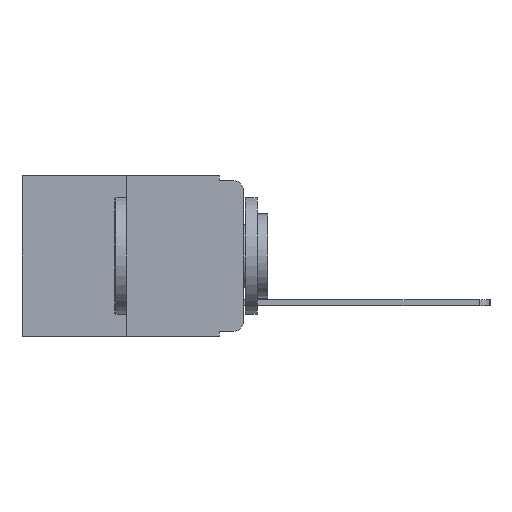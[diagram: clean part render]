
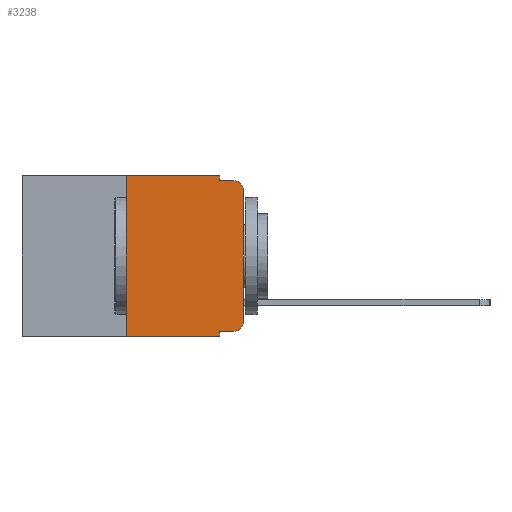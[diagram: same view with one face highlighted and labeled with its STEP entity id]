
A CAD part, left-side view. The second image highlights one B-rep face of the part: STEP entity #3238.
In plain terms, the highlighted planar face has unit normal (-1, 0, 0).
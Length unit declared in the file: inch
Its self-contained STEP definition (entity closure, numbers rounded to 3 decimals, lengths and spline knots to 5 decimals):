
#72 = ORIENTED_EDGE ( 'NONE', *, *, #2104, .F. ) ;
#92 = EDGE_CURVE ( 'NONE', #22968, #7479, #22821, .T. ) ;
#195 = VECTOR ( 'NONE', #9870, 39.37008 ) ;
#472 = DIRECTION ( 'NONE',  ( 0., -1., 0. ) ) ;
#510 = CIRCLE ( 'NONE', #16154, 0.02 ) ;
#915 = EDGE_CURVE ( 'NONE', #16615, #19250, #18439, .T. ) ;
#943 = CARTESIAN_POINT ( 'NONE',  ( 0., 0.25, 0. ) ) ;
#1352 = VERTEX_POINT ( 'NONE', #4210 ) ;
#1891 = AXIS2_PLACEMENT_3D ( 'NONE', #5693, #5776, #18304 ) ;
#2012 = ORIENTED_EDGE ( 'NONE', *, *, #2025, .T. ) ;
#2025 = EDGE_CURVE ( 'NONE', #11673, #21753, #6939, .T. ) ;
#2029 = EDGE_CURVE ( 'NONE', #21753, #4110, #510, .T. ) ;
#2096 = EDGE_CURVE ( 'NONE', #11606, #4110, #17285, .T. ) ;
#2104 = EDGE_CURVE ( 'NONE', #19250, #11606, #2763, .T. ) ;
#2208 = EDGE_CURVE ( 'NONE', #22968, #16615, #4902, .T. ) ;
#2303 = ORIENTED_EDGE ( 'NONE', *, *, #2434, .T. ) ;
#2334 = EDGE_CURVE ( 'NONE', #21268, #7479, #16415, .T. ) ;
#2406 = EDGE_CURVE ( 'NONE', #21268, #1352, #9529, .T. ) ;
#2434 = EDGE_CURVE ( 'NONE', #1352, #11673, #13143, .T. ) ;
#2763 = LINE ( 'NONE', #9090, #16729 ) ;
#3238 = ADVANCED_FACE ( 'NONE', ( #14453 ), #12986, .F. ) ;
#3280 = CARTESIAN_POINT ( 'NONE',  ( 0., 0.051, -0.333 ) ) ;
#4050 = CARTESIAN_POINT ( 'NONE',  ( 0., 0.051, -0.01 ) ) ;
#4110 = VERTEX_POINT ( 'NONE', #19022 ) ;
#4210 = CARTESIAN_POINT ( 'NONE',  ( 0., 0.02, -0.333 ) ) ;
#4368 = CARTESIAN_POINT ( 'NONE',  ( 0., 0.25, -0.343 ) ) ;
#4619 = VECTOR ( 'NONE', #20987, 39.37008 ) ;
#4902 = LINE ( 'NONE', #9058, #195 ) ;
#5693 = CARTESIAN_POINT ( 'NONE',  ( 0., 0.473, 0. ) ) ;
#5776 = DIRECTION ( 'NONE',  ( 1., 0., 0. ) ) ;
#6029 = ORIENTED_EDGE ( 'NONE', *, *, #915, .F. ) ;
#6939 = LINE ( 'NONE', #19309, #19492 ) ;
#7479 = VERTEX_POINT ( 'NONE', #22051 ) ;
#7989 = ORIENTED_EDGE ( 'NONE', *, *, #2208, .F. ) ;
#8388 = VECTOR ( 'NONE', #472, 39.37008 ) ;
#8514 = DIRECTION ( 'NONE',  ( 0., 0., -1. ) ) ;
#8597 = CARTESIAN_POINT ( 'NONE',  ( 0., 0.051, 0. ) ) ;
#8920 = ORIENTED_EDGE ( 'NONE', *, *, #92, .T. ) ;
#9058 = CARTESIAN_POINT ( 'NONE',  ( 0., 0.25, 0. ) ) ;
#9090 = CARTESIAN_POINT ( 'NONE',  ( 0., 0.051, 0. ) ) ;
#9529 = LINE ( 'NONE', #20834, #4619 ) ;
#9870 = DIRECTION ( 'NONE',  ( 0., 0., 1. ) ) ;
#10594 = DIRECTION ( 'NONE',  ( 0., -1., 0. ) ) ;
#11568 = ORIENTED_EDGE ( 'NONE', *, *, #2334, .F. ) ;
#11606 = VERTEX_POINT ( 'NONE', #4050 ) ;
#11673 = VERTEX_POINT ( 'NONE', #20457 ) ;
#11766 = VECTOR ( 'NONE', #8514, 39.37008 ) ;
#11839 = CARTESIAN_POINT ( 'NONE',  ( 0., 0., -0.03 ) ) ;
#11984 = CARTESIAN_POINT ( 'NONE',  ( 0., 0.051, -0.01 ) ) ;
#12227 = DIRECTION ( 'NONE',  ( 0., 0., -1. ) ) ;
#12986 = PLANE ( 'NONE',  #1891 ) ;
#12996 = ORIENTED_EDGE ( 'NONE', *, *, #2406, .T. ) ;
#13143 = CIRCLE ( 'NONE', #15277, 0.02 ) ;
#13930 = DIRECTION ( 'NONE',  ( 0., 0., -1. ) ) ;
#13988 = DIRECTION ( 'NONE',  ( -1., 0., 0. ) ) ;
#14453 = FACE_OUTER_BOUND ( 'NONE', #14902, .T. ) ;
#14902 = EDGE_LOOP ( 'NONE', ( #2012, #19702, #20323, #72, #6029, #7989, #8920, #11568, #12996, #2303 ) ) ;
#15277 = AXIS2_PLACEMENT_3D ( 'NONE', #22834, #22789, #17047 ) ;
#15453 = CARTESIAN_POINT ( 'NONE',  ( 0., 0.02, -0.03 ) ) ;
#15555 = CARTESIAN_POINT ( 'NONE',  ( 0., 0.051, 0. ) ) ;
#15913 = DIRECTION ( 'NONE',  ( 0., -1., 0. ) ) ;
#16154 = AXIS2_PLACEMENT_3D ( 'NONE', #15453, #13988, #13930 ) ;
#16415 = LINE ( 'NONE', #8597, #11766 ) ;
#16471 = CARTESIAN_POINT ( 'NONE',  ( 0., 0.473, 0. ) ) ;
#16615 = VERTEX_POINT ( 'NONE', #943 ) ;
#16729 = VECTOR ( 'NONE', #12227, 39.37008 ) ;
#17047 = DIRECTION ( 'NONE',  ( 0., 0., -1. ) ) ;
#17285 = LINE ( 'NONE', #11984, #8388 ) ;
#17594 = DIRECTION ( 'NONE',  ( 0., 0., 1. ) ) ;
#18217 = VECTOR ( 'NONE', #10594, 39.37008 ) ;
#18303 = CARTESIAN_POINT ( 'NONE',  ( 0., 0.473, -0.343 ) ) ;
#18304 = DIRECTION ( 'NONE',  ( 0., 0., -1. ) ) ;
#18439 = LINE ( 'NONE', #16471, #22490 ) ;
#19022 = CARTESIAN_POINT ( 'NONE',  ( 0., 0.02, -0.01 ) ) ;
#19250 = VERTEX_POINT ( 'NONE', #15555 ) ;
#19309 = CARTESIAN_POINT ( 'NONE',  ( 0., 0., 0. ) ) ;
#19492 = VECTOR ( 'NONE', #17594, 39.37008 ) ;
#19702 = ORIENTED_EDGE ( 'NONE', *, *, #2029, .T. ) ;
#20323 = ORIENTED_EDGE ( 'NONE', *, *, #2096, .F. ) ;
#20457 = CARTESIAN_POINT ( 'NONE',  ( 0., 0., -0.313 ) ) ;
#20834 = CARTESIAN_POINT ( 'NONE',  ( 0., 0.051, -0.333 ) ) ;
#20987 = DIRECTION ( 'NONE',  ( 0., -1., 0. ) ) ;
#21268 = VERTEX_POINT ( 'NONE', #3280 ) ;
#21753 = VERTEX_POINT ( 'NONE', #11839 ) ;
#22051 = CARTESIAN_POINT ( 'NONE',  ( 0., 0.051, -0.343 ) ) ;
#22490 = VECTOR ( 'NONE', #15913, 39.37008 ) ;
#22789 = DIRECTION ( 'NONE',  ( -1., 0., 0. ) ) ;
#22821 = LINE ( 'NONE', #18303, #18217 ) ;
#22834 = CARTESIAN_POINT ( 'NONE',  ( 0., 0.02, -0.313 ) ) ;
#22968 = VERTEX_POINT ( 'NONE', #4368 ) ;
